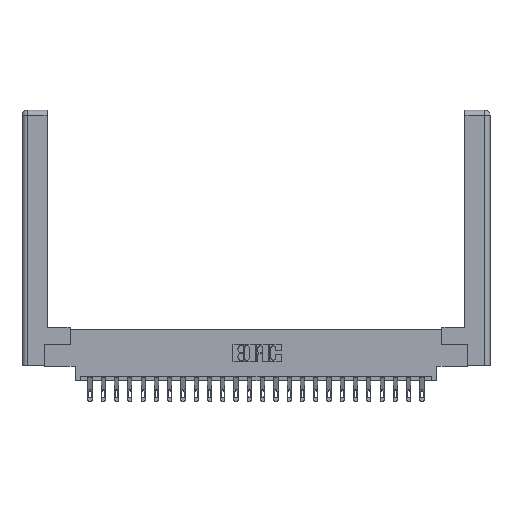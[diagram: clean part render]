
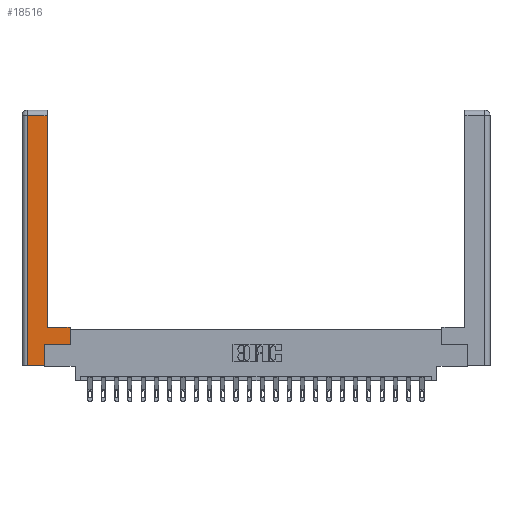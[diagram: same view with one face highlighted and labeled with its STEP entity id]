
A CAD part, top view. The second image highlights one B-rep face of the part: STEP entity #18516.
In plain terms, the highlighted planar face has unit normal (0, 0, 1).
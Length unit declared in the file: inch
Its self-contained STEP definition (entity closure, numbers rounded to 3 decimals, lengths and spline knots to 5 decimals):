
#338 = EDGE_CURVE ( 'NONE', #4716, #1841, #10639, .T. ) ;
#399 = EDGE_LOOP ( 'NONE', ( #471, #9356, #1863, #11985, #7329, #19430, #8828, #1587 ) ) ;
#471 = ORIENTED_EDGE ( 'NONE', *, *, #23310, .T. ) ;
#937 = DIRECTION ( 'NONE',  ( 0., 1., 0. ) ) ;
#1146 = VERTEX_POINT ( 'NONE', #23031 ) ;
#1184 = VECTOR ( 'NONE', #24231, 39.37008 ) ;
#1277 = CARTESIAN_POINT ( 'NONE',  ( 0.265, 0., 0. ) ) ;
#1557 = PLANE ( 'NONE',  #10054 ) ;
#1587 = ORIENTED_EDGE ( 'NONE', *, *, #3934, .T. ) ;
#1815 = LINE ( 'NONE', #14320, #1184 ) ;
#1841 = VERTEX_POINT ( 'NONE', #22188 ) ;
#1863 = ORIENTED_EDGE ( 'NONE', *, *, #338, .T. ) ;
#1890 = CARTESIAN_POINT ( 'NONE',  ( 0., 0., 0. ) ) ;
#2113 = LINE ( 'NONE', #24260, #18663 ) ;
#2569 = CARTESIAN_POINT ( 'NONE',  ( 0.565, 0.245, 0. ) ) ;
#3018 = LINE ( 'NONE', #24770, #21428 ) ;
#3847 = CARTESIAN_POINT ( 'NONE',  ( 0.0615, 2.94, 0. ) ) ;
#3934 = EDGE_CURVE ( 'NONE', #3944, #21238, #8772, .T. ) ;
#3944 = VERTEX_POINT ( 'NONE', #20483 ) ;
#4117 = VERTEX_POINT ( 'NONE', #2569 ) ;
#4716 = VERTEX_POINT ( 'NONE', #22422 ) ;
#6697 = VECTOR ( 'NONE', #16377, 39.37008 ) ;
#6865 = DIRECTION ( 'NONE',  ( -1., 0., 0. ) ) ;
#7329 = ORIENTED_EDGE ( 'NONE', *, *, #23626, .T. ) ;
#7588 = VECTOR ( 'NONE', #17267, 39.37008 ) ;
#8772 = LINE ( 'NONE', #14690, #23840 ) ;
#8828 = ORIENTED_EDGE ( 'NONE', *, *, #22122, .T. ) ;
#9356 = ORIENTED_EDGE ( 'NONE', *, *, #24080, .T. ) ;
#9584 = EDGE_CURVE ( 'NONE', #1841, #14905, #20425, .T. ) ;
#10054 = AXIS2_PLACEMENT_3D ( 'NONE', #1890, #17200, #13342 ) ;
#10204 = CARTESIAN_POINT ( 'NONE',  ( 0.265, 0.245, 0. ) ) ;
#10639 = LINE ( 'NONE', #24224, #6697 ) ;
#10706 = DIRECTION ( 'NONE',  ( 0., 1., 0. ) ) ;
#11718 = FACE_OUTER_BOUND ( 'NONE', #399, .T. ) ;
#11985 = ORIENTED_EDGE ( 'NONE', *, *, #9584, .T. ) ;
#12311 = DIRECTION ( 'NONE',  ( 0., 1., 0. ) ) ;
#13342 = DIRECTION ( 'NONE',  ( -1., 0., 0. ) ) ;
#14320 = CARTESIAN_POINT ( 'NONE',  ( 0.565, 0.245, 0. ) ) ;
#14398 = LINE ( 'NONE', #22057, #19660 ) ;
#14690 = CARTESIAN_POINT ( 'NONE',  ( 0.295, 0.45, 0. ) ) ;
#14905 = VERTEX_POINT ( 'NONE', #1277 ) ;
#15969 = CARTESIAN_POINT ( 'NONE',  ( 0.295, 0.45, 0. ) ) ;
#16377 = DIRECTION ( 'NONE',  ( 0., -1., 0. ) ) ;
#16607 = CARTESIAN_POINT ( 'NONE',  ( 0.265, 0., 0. ) ) ;
#17200 = DIRECTION ( 'NONE',  ( 0., 0., -1. ) ) ;
#17267 = DIRECTION ( 'NONE',  ( -1., 0., 0. ) ) ;
#17553 = VERTEX_POINT ( 'NONE', #10204 ) ;
#18516 = ADVANCED_FACE ( 'NONE', ( #11718 ), #1557, .F. ) ;
#18663 = VECTOR ( 'NONE', #937, 39.37008 ) ;
#19430 = ORIENTED_EDGE ( 'NONE', *, *, #23537, .T. ) ;
#19660 = VECTOR ( 'NONE', #12311, 39.37008 ) ;
#20251 = DIRECTION ( 'NONE',  ( 1., 0., 0. ) ) ;
#20425 = LINE ( 'NONE', #16607, #23510 ) ;
#20483 = CARTESIAN_POINT ( 'NONE',  ( 0.565, 0.45, 0. ) ) ;
#21238 = VERTEX_POINT ( 'NONE', #15969 ) ;
#21428 = VECTOR ( 'NONE', #10706, 39.37008 ) ;
#22057 = CARTESIAN_POINT ( 'NONE',  ( 0.565, 0.45, 0. ) ) ;
#22122 = EDGE_CURVE ( 'NONE', #4117, #3944, #14398, .T. ) ;
#22188 = CARTESIAN_POINT ( 'NONE',  ( 0.0615, 0., 0. ) ) ;
#22422 = CARTESIAN_POINT ( 'NONE',  ( 0.0615, 2.94, 0. ) ) ;
#23031 = CARTESIAN_POINT ( 'NONE',  ( 0.295, 2.94, 0. ) ) ;
#23310 = EDGE_CURVE ( 'NONE', #21238, #1146, #2113, .T. ) ;
#23510 = VECTOR ( 'NONE', #20251, 39.37008 ) ;
#23537 = EDGE_CURVE ( 'NONE', #17553, #4117, #1815, .T. ) ;
#23626 = EDGE_CURVE ( 'NONE', #14905, #17553, #3018, .T. ) ;
#23840 = VECTOR ( 'NONE', #6865, 39.37008 ) ;
#23848 = LINE ( 'NONE', #3847, #7588 ) ;
#24080 = EDGE_CURVE ( 'NONE', #1146, #4716, #23848, .T. ) ;
#24224 = CARTESIAN_POINT ( 'NONE',  ( 0.0615, 0., 0. ) ) ;
#24231 = DIRECTION ( 'NONE',  ( 1., 0., 0. ) ) ;
#24260 = CARTESIAN_POINT ( 'NONE',  ( 0.295, 3., 0. ) ) ;
#24770 = CARTESIAN_POINT ( 'NONE',  ( 0.265, 0.245, 0. ) ) ;
